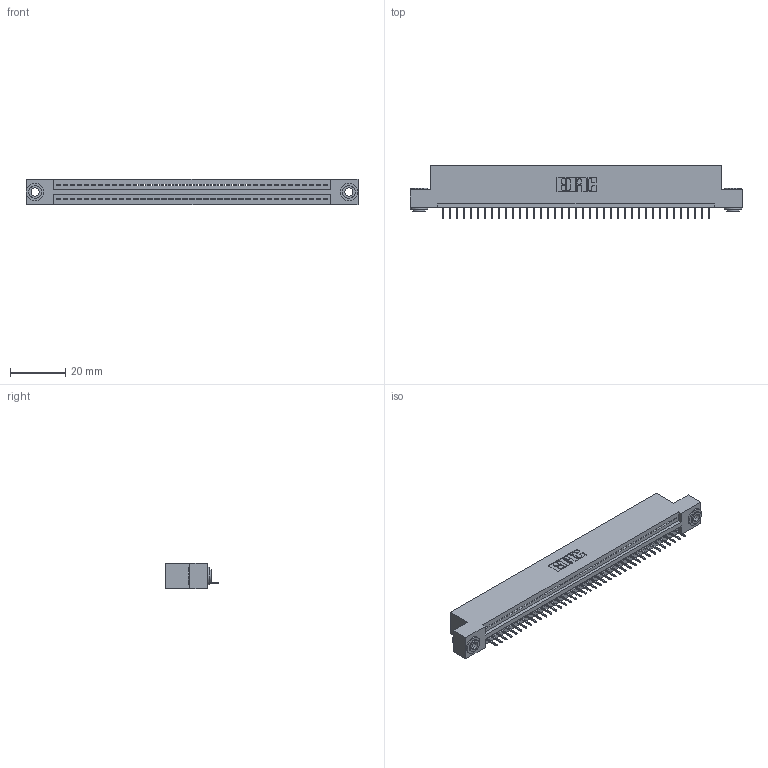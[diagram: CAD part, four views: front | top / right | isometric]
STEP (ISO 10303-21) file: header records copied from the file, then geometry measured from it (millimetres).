
FILE_DESCRIPTION (( 'STEP AP203' ), '1' );
FILE_NAME ('345-039-524-103.STEP', '2019-10-08T06:13:42', ( '' ), ( '' ), 'SwSTEP 2.0', 'SolidWorks 2016', '' );
FILE_SCHEMA (( 'CONFIG_CONTROL_DESIGN' ));
Length unit declared in the file: inch
Products named in the file (4): 345 Part_Flush Mounting Lugs - 0.156 Dia-TH; 345-292-001_345-293-124; 345-039-524-103; 345-250-002_345-250-002-102
Assembly tree (42 placements, depth 2):
  345-039-524-103
    345 Part_Flush Mounting Lugs - 0.156 Dia-TH
    345-292-001_345-293-124  x39
    345-250-002_345-250-002-102  x2
Bounding box: 120.27 x 19.35 x 9.4 mm (x, y, z)
Volume: 11264 mm3; surface area: 14650 mm2
Topology: 42 solids, 42 shells, 2582 faces, 7437 edges, 4798 vertices
Faces by surface type: plane 1884, cylinder 690, cone 8
Entity records: 30480 total; most frequent: CARTESIAN_POINT 5256, ORIENTED_EDGE 5222, DIRECTION 4627, EDGE_CURVE 2611, LINE 2303, VECTOR 2303, VERTEX_POINT 1734, AXIS2_PLACEMENT_3D 1162
